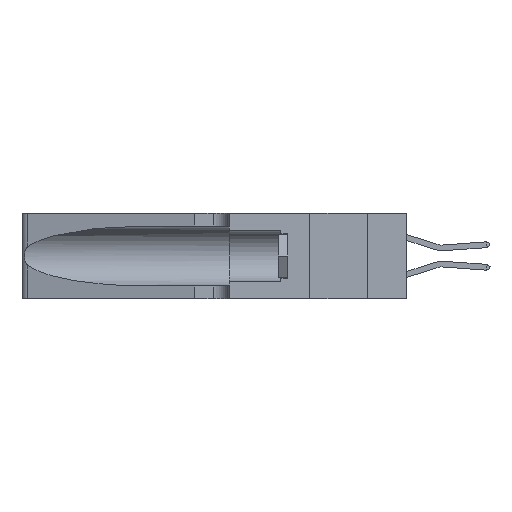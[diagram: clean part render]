
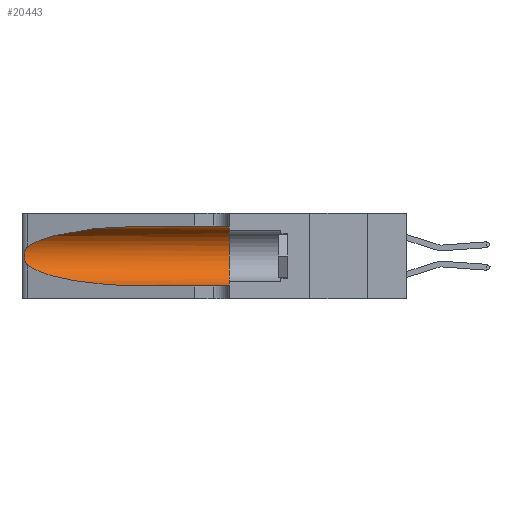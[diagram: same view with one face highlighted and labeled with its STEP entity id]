
A CAD part, left-side view. The second image highlights one B-rep face of the part: STEP entity #20443.
In plain terms, the highlighted cylindrical face has radius 3.308 mm (diameter 6.617 mm), a partial arc.
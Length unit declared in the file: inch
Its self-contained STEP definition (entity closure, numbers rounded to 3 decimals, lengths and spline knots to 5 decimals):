
#822 = CARTESIAN_POINT ( 'NONE',  ( 0.25487, 1.22718, 0.14631 ) ) ;
#2247 = EDGE_CURVE ( 'NONE', #28864, #8683, #25871, .T. ) ;
#2410 =( BOUNDED_CURVE ( )  B_SPLINE_CURVE ( 3, ( #19360, #24551, #15439, #10866 ),
 .UNSPECIFIED., .F., .F. ) 
 B_SPLINE_CURVE_WITH_KNOTS ( ( 4, 4 ),
 ( 1.5708, 2.84003 ),
 .UNSPECIFIED. ) 
 CURVE ( )  GEOMETRIC_REPRESENTATION_ITEM ( )  RATIONAL_B_SPLINE_CURVE ( ( 1., 0.87, 0.87, 1. ) ) 
 REPRESENTATION_ITEM ( '' )  );
#2850 = CARTESIAN_POINT ( 'NONE',  ( 0.26017, 1.23833, 0.17102 ) ) ;
#3156 = CARTESIAN_POINT ( 'NONE',  ( 0.25639, 1.23186, 0.15144 ) ) ;
#3394 = EDGE_CURVE ( 'NONE', #17216, #25916, #7253, .T. ) ;
#3650 = ORIENTED_EDGE ( 'NONE', *, *, #16654, .T. ) ;
#3991 = CARTESIAN_POINT ( 'NONE',  ( 0.1305, 0.35, 0.31525 ) ) ;
#4108 = CARTESIAN_POINT ( 'NONE',  ( 0.2373, 1.15595, 0.08982 ) ) ;
#5108 = CARTESIAN_POINT ( 'NONE',  ( 0.25787, 1.23484, 0.2124 ) ) ;
#5598 = CARTESIAN_POINT ( 'NONE',  ( 0.1305, 1.61858, 0.31525 ) ) ;
#5973 = CYLINDRICAL_SURFACE ( 'NONE', #14258, 0.13025 ) ;
#7253 = LINE ( 'NONE', #15760, #30272 ) ;
#8670 = EDGE_CURVE ( 'NONE', #23733, #17216, #16381, .T. ) ;
#8683 = VERTEX_POINT ( 'NONE', #3991 ) ;
#9689 = VECTOR ( 'NONE', #20894, 39.37008 ) ;
#10122 = VERTEX_POINT ( 'NONE', #11431 ) ;
#10403 = CARTESIAN_POINT ( 'NONE',  ( 0.25856, 1.23593, 0.16098 ) ) ;
#10866 = CARTESIAN_POINT ( 'NONE',  ( 0.25487, 1.22718, 0.22369 ) ) ;
#11431 = CARTESIAN_POINT ( 'NONE',  ( 0.25487, 1.22718, 0.22369 ) ) ;
#11766 = ORIENTED_EDGE ( 'NONE', *, *, #2247, .F. ) ;
#11863 = B_SPLINE_CURVE_WITH_KNOTS ( 'NONE', 3,
 ( #20021, #20262, #20996, #5108, #20590, #15679, #28369, #31075, #2850, #10403, #12883, #3156, #18807, #822 ),
 .UNSPECIFIED., .F., .F.,
 ( 4, 2, 2, 2, 2, 2, 4 ),
 ( 0., 0.00027, 0.00053, 0.00107, 0.0016, 0.00187, 0.00214 ),
 .UNSPECIFIED. ) ;
#12883 = CARTESIAN_POINT ( 'NONE',  ( 0.25789, 1.23486, 0.15765 ) ) ;
#13184 = ORIENTED_EDGE ( 'NONE', *, *, #8670, .T. ) ;
#13577 = DIRECTION ( 'NONE',  ( 0., -1., 0. ) ) ;
#13656 = DIRECTION ( 'NONE',  ( 0., 1., 0. ) ) ;
#14034 = EDGE_CURVE ( 'NONE', #10122, #23733, #11863, .T. ) ;
#14226 = CARTESIAN_POINT ( 'NONE',  ( 0.18966, 0.96281, 0.05475 ) ) ;
#14258 = AXIS2_PLACEMENT_3D ( 'NONE', #16528, #21621, #17140 ) ;
#15046 = EDGE_LOOP ( 'NONE', ( #3650, #19522, #13184, #30922, #16511, #11766 ) ) ;
#15283 = CARTESIAN_POINT ( 'NONE',  ( 0.1305, 0.72297, 0.05475 ) ) ;
#15439 = CARTESIAN_POINT ( 'NONE',  ( 0.2373, 1.15595, 0.28018 ) ) ;
#15679 = CARTESIAN_POINT ( 'NONE',  ( 0.26018, 1.23835, 0.19895 ) ) ;
#15760 = CARTESIAN_POINT ( 'NONE',  ( 0.1305, 1.61858, 0.05475 ) ) ;
#16270 = CARTESIAN_POINT ( 'NONE',  ( 0.1305, 0.35, 0.185 ) ) ;
#16271 = AXIS2_PLACEMENT_3D ( 'NONE', #16270, #13656, #24068 ) ;
#16381 =( BOUNDED_CURVE ( )  B_SPLINE_CURVE ( 3, ( #24868, #4108, #14226, #32426 ),
 .UNSPECIFIED., .F., .T. ) 
 B_SPLINE_CURVE_WITH_KNOTS ( ( 4, 4 ),
 ( 3.44316, 4.71239 ),
 .UNSPECIFIED. ) 
 CURVE ( )  GEOMETRIC_REPRESENTATION_ITEM ( )  RATIONAL_B_SPLINE_CURVE ( ( 1., 0.87, 0.87, 1. ) ) 
 REPRESENTATION_ITEM ( '' )  );
#16511 = ORIENTED_EDGE ( 'NONE', *, *, #25046, .F. ) ;
#16528 = CARTESIAN_POINT ( 'NONE',  ( 0.1305, 1.61858, 0.185 ) ) ;
#16654 = EDGE_CURVE ( 'NONE', #28864, #10122, #2410, .T. ) ;
#17140 = DIRECTION ( 'NONE',  ( 0., 0., -1. ) ) ;
#17216 = VERTEX_POINT ( 'NONE', #15283 ) ;
#18807 = CARTESIAN_POINT ( 'NONE',  ( 0.25555, 1.22993, 0.14849 ) ) ;
#19360 = CARTESIAN_POINT ( 'NONE',  ( 0.1305, 0.72297, 0.31525 ) ) ;
#19522 = ORIENTED_EDGE ( 'NONE', *, *, #14034, .T. ) ;
#20021 = CARTESIAN_POINT ( 'NONE',  ( 0.25487, 1.22718, 0.22369 ) ) ;
#20262 = CARTESIAN_POINT ( 'NONE',  ( 0.25555, 1.22994, 0.2215 ) ) ;
#20443 = ADVANCED_FACE ( 'NONE', ( #24177 ), #5973, .F. ) ;
#20590 = CARTESIAN_POINT ( 'NONE',  ( 0.25854, 1.2359, 0.20912 ) ) ;
#20894 = DIRECTION ( 'NONE',  ( 0., -1., 0. ) ) ;
#20996 = CARTESIAN_POINT ( 'NONE',  ( 0.25639, 1.23184, 0.21858 ) ) ;
#21599 = CARTESIAN_POINT ( 'NONE',  ( 0.25487, 1.22718, 0.14631 ) ) ;
#21621 = DIRECTION ( 'NONE',  ( 0., -1., 0. ) ) ;
#23733 = VERTEX_POINT ( 'NONE', #21599 ) ;
#24068 = DIRECTION ( 'NONE',  ( 0., 0., 1. ) ) ;
#24177 = FACE_OUTER_BOUND ( 'NONE', #15046, .T. ) ;
#24551 = CARTESIAN_POINT ( 'NONE',  ( 0.18966, 0.96281, 0.31525 ) ) ;
#24868 = CARTESIAN_POINT ( 'NONE',  ( 0.25487, 1.22718, 0.14631 ) ) ;
#25046 = EDGE_CURVE ( 'NONE', #8683, #25916, #33272, .T. ) ;
#25871 = LINE ( 'NONE', #5598, #9689 ) ;
#25916 = VERTEX_POINT ( 'NONE', #26856 ) ;
#26856 = CARTESIAN_POINT ( 'NONE',  ( 0.1305, 0.35, 0.05475 ) ) ;
#28349 = CARTESIAN_POINT ( 'NONE',  ( 0.1305, 0.72297, 0.31525 ) ) ;
#28369 = CARTESIAN_POINT ( 'NONE',  ( 0.26075, 1.23896, 0.19203 ) ) ;
#28864 = VERTEX_POINT ( 'NONE', #28349 ) ;
#30272 = VECTOR ( 'NONE', #13577, 39.37008 ) ;
#30922 = ORIENTED_EDGE ( 'NONE', *, *, #3394, .T. ) ;
#31075 = CARTESIAN_POINT ( 'NONE',  ( 0.26075, 1.23896, 0.178 ) ) ;
#32426 = CARTESIAN_POINT ( 'NONE',  ( 0.1305, 0.72297, 0.05475 ) ) ;
#33272 = CIRCLE ( 'NONE', #16271, 0.13025 ) ;
